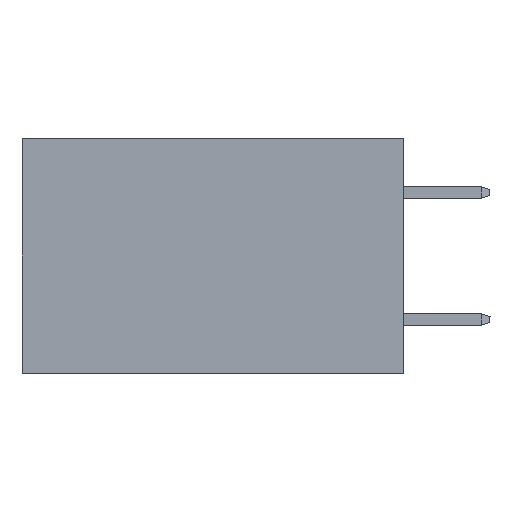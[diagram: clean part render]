
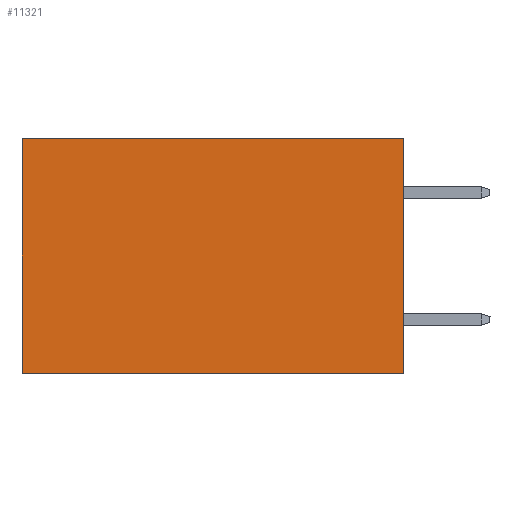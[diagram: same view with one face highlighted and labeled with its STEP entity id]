
A CAD part, left-side view. The second image highlights one B-rep face of the part: STEP entity #11321.
In plain terms, the highlighted planar face has unit normal (-1, 0, 0).
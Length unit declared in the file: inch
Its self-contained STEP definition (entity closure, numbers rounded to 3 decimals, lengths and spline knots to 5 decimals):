
#35 = CARTESIAN_POINT ( 'NONE',  ( 0.2875, 0., 0. ) ) ;
#688 = VERTEX_POINT ( 'NONE', #17987 ) ;
#1361 = CARTESIAN_POINT ( 'NONE',  ( 0.2875, 0.6, 0. ) ) ;
#2088 = CARTESIAN_POINT ( 'NONE',  ( 0.2875, 0., -0.37 ) ) ;
#2101 = ORIENTED_EDGE ( 'NONE', *, *, #5259, .T. ) ;
#2234 = VECTOR ( 'NONE', #11743, 39.37008 ) ;
#2251 = EDGE_CURVE ( 'NONE', #688, #13799, #7497, .T. ) ;
#3232 = ORIENTED_EDGE ( 'NONE', *, *, #2251, .T. ) ;
#3561 = CARTESIAN_POINT ( 'NONE',  ( 0.2875, 0., 0. ) ) ;
#3656 = LINE ( 'NONE', #3561, #18195 ) ;
#3785 = DIRECTION ( 'NONE',  ( 0., 1., 0. ) ) ;
#4145 = PLANE ( 'NONE',  #10657 ) ;
#4329 = DIRECTION ( 'NONE',  ( 0., 0., -1. ) ) ;
#4468 = EDGE_CURVE ( 'NONE', #688, #16753, #3656, .T. ) ;
#5259 = EDGE_CURVE ( 'NONE', #13799, #11976, #11674, .T. ) ;
#5729 = DIRECTION ( 'NONE',  ( 1., 0., 0. ) ) ;
#7497 = LINE ( 'NONE', #13535, #2234 ) ;
#8035 = ORIENTED_EDGE ( 'NONE', *, *, #4468, .F. ) ;
#9206 = LINE ( 'NONE', #2088, #12471 ) ;
#9243 = CARTESIAN_POINT ( 'NONE',  ( 0.2875, 0., -0.37 ) ) ;
#9690 = CARTESIAN_POINT ( 'NONE',  ( 0.2875, 0.6, -0.37 ) ) ;
#10657 = AXIS2_PLACEMENT_3D ( 'NONE', #35, #5729, #4329 ) ;
#11274 = FACE_OUTER_BOUND ( 'NONE', #13853, .T. ) ;
#11321 = ADVANCED_FACE ( 'NONE', ( #11274 ), #4145, .F. ) ;
#11674 = LINE ( 'NONE', #1361, #18224 ) ;
#11743 = DIRECTION ( 'NONE',  ( 0., 1., 0. ) ) ;
#11976 = VERTEX_POINT ( 'NONE', #9690 ) ;
#12090 = DIRECTION ( 'NONE',  ( 0., 0., -1. ) ) ;
#12385 = ORIENTED_EDGE ( 'NONE', *, *, #15831, .F. ) ;
#12471 = VECTOR ( 'NONE', #3785, 39.37008 ) ;
#12829 = DIRECTION ( 'NONE',  ( 0., 0., -1. ) ) ;
#13535 = CARTESIAN_POINT ( 'NONE',  ( 0.2875, 0., 0. ) ) ;
#13799 = VERTEX_POINT ( 'NONE', #14318 ) ;
#13853 = EDGE_LOOP ( 'NONE', ( #2101, #12385, #8035, #3232 ) ) ;
#14318 = CARTESIAN_POINT ( 'NONE',  ( 0.2875, 0.6, 0. ) ) ;
#15831 = EDGE_CURVE ( 'NONE', #16753, #11976, #9206, .T. ) ;
#16753 = VERTEX_POINT ( 'NONE', #9243 ) ;
#17987 = CARTESIAN_POINT ( 'NONE',  ( 0.2875, 0., 0. ) ) ;
#18195 = VECTOR ( 'NONE', #12090, 39.37008 ) ;
#18224 = VECTOR ( 'NONE', #12829, 39.37008 ) ;
